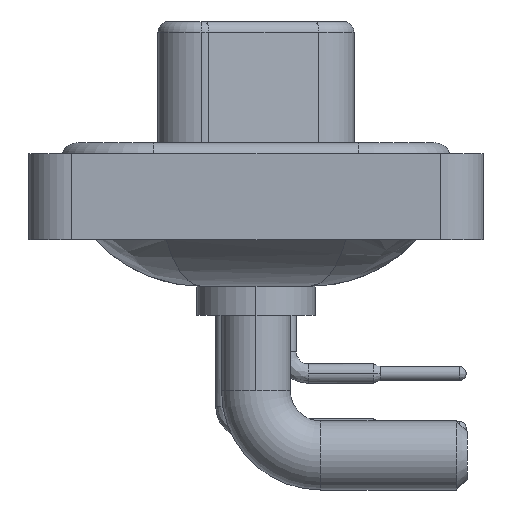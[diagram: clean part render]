
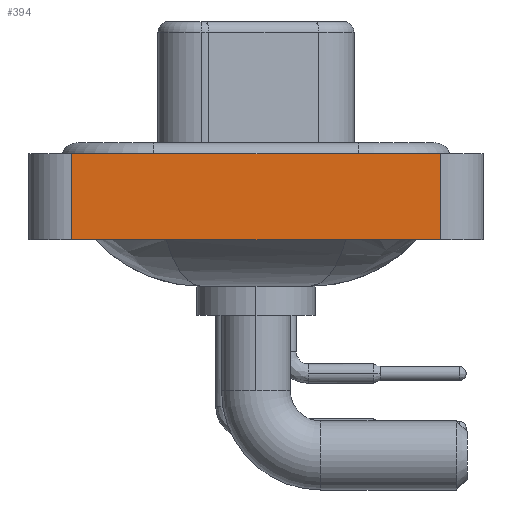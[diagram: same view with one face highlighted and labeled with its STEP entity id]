
A CAD part, left-side view. The second image highlights one B-rep face of the part: STEP entity #394.
In plain terms, the highlighted planar face has unit normal (-1, 0, 0).
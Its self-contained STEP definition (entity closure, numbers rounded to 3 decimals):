
#224 = LINE ( 'NONE', #4741, #15125 ) ;
#340 = DIRECTION ( 'NONE',  ( 0., 0., 1. ) ) ;
#394 = ADVANCED_FACE ( 'NONE', ( #22588 ), #2479, .T. ) ;
#740 = LINE ( 'NONE', #10705, #3705 ) ;
#1701 = VECTOR ( 'NONE', #340, 1000. ) ;
#2180 = LINE ( 'NONE', #18346, #5112 ) ;
#2479 = PLANE ( 'NONE',  #16658 ) ;
#2759 = CARTESIAN_POINT ( 'NONE',  ( -7.35, -8.55, 0.4 ) ) ;
#3433 = VERTEX_POINT ( 'NONE', #9535 ) ;
#3705 = VECTOR ( 'NONE', #8446, 1000. ) ;
#4741 = CARTESIAN_POINT ( 'NONE',  ( -7.35, -8.55, -3.6 ) ) ;
#4990 = LINE ( 'NONE', #18496, #1701 ) ;
#5112 = VECTOR ( 'NONE', #13856, 1000. ) ;
#6844 = DIRECTION ( 'NONE',  ( 0., 0., 1. ) ) ;
#6968 = DIRECTION ( 'NONE',  ( -1., 0., 0. ) ) ;
#7232 = EDGE_CURVE ( 'NONE', #21652, #22361, #2180, .T. ) ;
#7541 = CARTESIAN_POINT ( 'NONE',  ( -7.35, -8.55, -3.6 ) ) ;
#8446 = DIRECTION ( 'NONE',  ( 0., -1., 0. ) ) ;
#8753 = ORIENTED_EDGE ( 'NONE', *, *, #19713, .T. ) ;
#9535 = CARTESIAN_POINT ( 'NONE',  ( -7.35, 8.55, -3.6 ) ) ;
#10564 = DIRECTION ( 'NONE',  ( 0., 0., 1. ) ) ;
#10705 = CARTESIAN_POINT ( 'NONE',  ( -7.35, -8.55, -3.6 ) ) ;
#12431 = CARTESIAN_POINT ( 'NONE',  ( -7.35, -8.55, -3.6 ) ) ;
#13593 = CARTESIAN_POINT ( 'NONE',  ( -7.35, 8.55, 0.4 ) ) ;
#13856 = DIRECTION ( 'NONE',  ( 0., -1., 0. ) ) ;
#15125 = VECTOR ( 'NONE', #6844, 1000. ) ;
#15939 = EDGE_CURVE ( 'NONE', #3433, #21652, #4990, .T. ) ;
#16658 = AXIS2_PLACEMENT_3D ( 'NONE', #12431, #6968, #10564 ) ;
#18346 = CARTESIAN_POINT ( 'NONE',  ( -7.35, -8.55, 0.4 ) ) ;
#18496 = CARTESIAN_POINT ( 'NONE',  ( -7.35, 8.55, -3.6 ) ) ;
#19705 = EDGE_CURVE ( 'NONE', #20676, #22361, #224, .T. ) ;
#19713 = EDGE_CURVE ( 'NONE', #3433, #20676, #740, .T. ) ;
#20676 = VERTEX_POINT ( 'NONE', #7541 ) ;
#20747 = ORIENTED_EDGE ( 'NONE', *, *, #15939, .F. ) ;
#21210 = ORIENTED_EDGE ( 'NONE', *, *, #19705, .T. ) ;
#21372 = EDGE_LOOP ( 'NONE', ( #21210, #23673, #20747, #8753 ) ) ;
#21652 = VERTEX_POINT ( 'NONE', #13593 ) ;
#22361 = VERTEX_POINT ( 'NONE', #2759 ) ;
#22588 = FACE_OUTER_BOUND ( 'NONE', #21372, .T. ) ;
#23673 = ORIENTED_EDGE ( 'NONE', *, *, #7232, .F. ) ;
